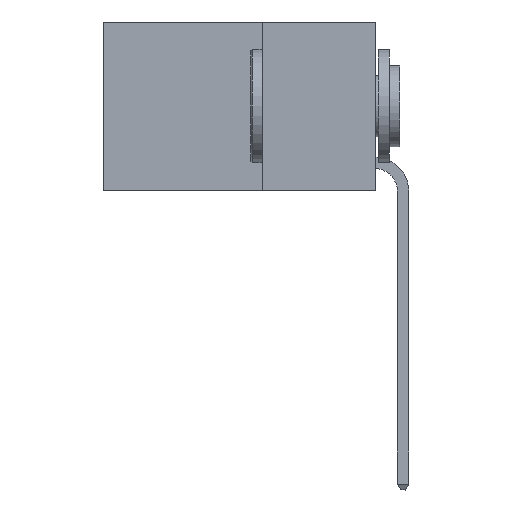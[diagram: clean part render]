
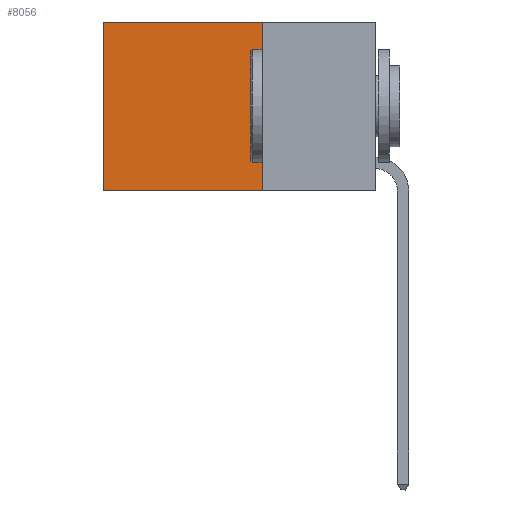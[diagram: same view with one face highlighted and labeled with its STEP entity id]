
A CAD part, left-side view. The second image highlights one B-rep face of the part: STEP entity #8056.
In plain terms, the highlighted planar face has unit normal (-1, 0, 0).
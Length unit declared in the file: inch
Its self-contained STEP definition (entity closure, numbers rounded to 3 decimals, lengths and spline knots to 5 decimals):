
#86 = LINE ( 'NONE', #2288, #8234 ) ;
#362 = ORIENTED_EDGE ( 'NONE', *, *, #11929, .F. ) ;
#512 = EDGE_CURVE ( 'NONE', #5226, #4465, #1257, .T. ) ;
#695 = EDGE_CURVE ( 'NONE', #4036, #8859, #11424, .T. ) ;
#827 = DIRECTION ( 'NONE',  ( 0., 1., 0. ) ) ;
#975 = CARTESIAN_POINT ( 'NONE',  ( 0.2625, 0.25, 0. ) ) ;
#1237 = FACE_OUTER_BOUND ( 'NONE', #1859, .T. ) ;
#1257 = LINE ( 'NONE', #2323, #10989 ) ;
#1859 = EDGE_LOOP ( 'NONE', ( #10852, #8085, #362, #10577 ) ) ;
#2288 = CARTESIAN_POINT ( 'NONE',  ( 0.2625, 0.6, 0. ) ) ;
#2323 = CARTESIAN_POINT ( 'NONE',  ( 0.2625, 0.25, -0.37 ) ) ;
#2529 = CARTESIAN_POINT ( 'NONE',  ( 0.2625, 0.25, 0. ) ) ;
#3031 = DIRECTION ( 'NONE',  ( 0., 0., -1. ) ) ;
#3834 = DIRECTION ( 'NONE',  ( 0., 0., -1. ) ) ;
#3920 = VECTOR ( 'NONE', #827, 39.37008 ) ;
#4036 = VERTEX_POINT ( 'NONE', #2529 ) ;
#4465 = VERTEX_POINT ( 'NONE', #8757 ) ;
#5226 = VERTEX_POINT ( 'NONE', #7997 ) ;
#5853 = PLANE ( 'NONE',  #6236 ) ;
#6236 = AXIS2_PLACEMENT_3D ( 'NONE', #6815, #8709, #3031 ) ;
#6308 = LINE ( 'NONE', #975, #8525 ) ;
#6337 = CARTESIAN_POINT ( 'NONE',  ( 0.2625, 0.25, 0. ) ) ;
#6815 = CARTESIAN_POINT ( 'NONE',  ( 0.2625, 0.25, 0. ) ) ;
#7095 = CARTESIAN_POINT ( 'NONE',  ( 0.2625, 0.6, 0. ) ) ;
#7302 = DIRECTION ( 'NONE',  ( 0., 1., 0. ) ) ;
#7997 = CARTESIAN_POINT ( 'NONE',  ( 0.2625, 0.25, -0.37 ) ) ;
#8056 = ADVANCED_FACE ( 'NONE', ( #1237 ), #5853, .F. ) ;
#8085 = ORIENTED_EDGE ( 'NONE', *, *, #512, .F. ) ;
#8234 = VECTOR ( 'NONE', #11665, 39.37008 ) ;
#8525 = VECTOR ( 'NONE', #3834, 39.37008 ) ;
#8709 = DIRECTION ( 'NONE',  ( 1., 0., 0. ) ) ;
#8757 = CARTESIAN_POINT ( 'NONE',  ( 0.2625, 0.6, -0.37 ) ) ;
#8859 = VERTEX_POINT ( 'NONE', #7095 ) ;
#10577 = ORIENTED_EDGE ( 'NONE', *, *, #695, .T. ) ;
#10852 = ORIENTED_EDGE ( 'NONE', *, *, #11427, .T. ) ;
#10989 = VECTOR ( 'NONE', #7302, 39.37008 ) ;
#11424 = LINE ( 'NONE', #6337, #3920 ) ;
#11427 = EDGE_CURVE ( 'NONE', #8859, #4465, #86, .T. ) ;
#11665 = DIRECTION ( 'NONE',  ( 0., 0., -1. ) ) ;
#11929 = EDGE_CURVE ( 'NONE', #4036, #5226, #6308, .T. ) ;
